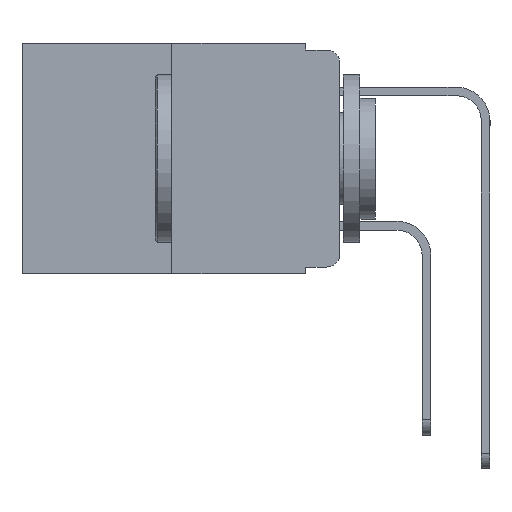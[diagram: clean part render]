
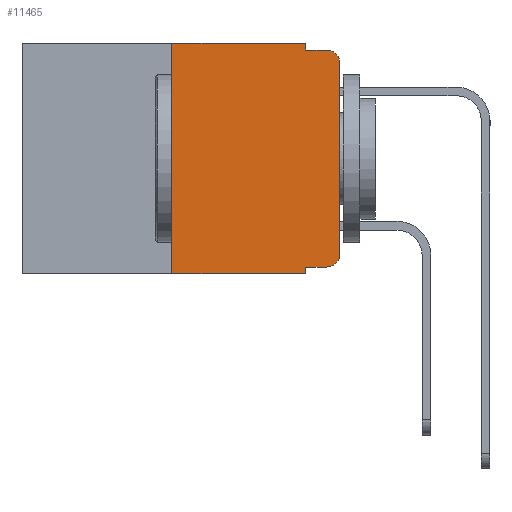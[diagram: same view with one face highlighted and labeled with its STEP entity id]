
A CAD part, left-side view. The second image highlights one B-rep face of the part: STEP entity #11465.
In plain terms, the highlighted planar face has unit normal (-1, 0, 0).
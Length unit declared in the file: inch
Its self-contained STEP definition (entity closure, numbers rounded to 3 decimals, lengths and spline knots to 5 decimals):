
#160 = CIRCLE ( 'NONE', #3296, 0.02 ) ;
#465 = LINE ( 'NONE', #10963, #16207 ) ;
#964 = VECTOR ( 'NONE', #10694, 39.37008 ) ;
#1460 = DIRECTION ( 'NONE',  ( 0., 0., -1. ) ) ;
#1743 = CARTESIAN_POINT ( 'NONE',  ( 0., 0.25, -0.343 ) ) ;
#1821 = ORIENTED_EDGE ( 'NONE', *, *, #17455, .T. ) ;
#2290 = CARTESIAN_POINT ( 'NONE',  ( 0., 0.051, -0.01 ) ) ;
#2610 = DIRECTION ( 'NONE',  ( -1., 0., 0. ) ) ;
#2672 = CARTESIAN_POINT ( 'NONE',  ( 0., 0.051, 0. ) ) ;
#2952 = VECTOR ( 'NONE', #3885, 39.37008 ) ;
#3296 = AXIS2_PLACEMENT_3D ( 'NONE', #12593, #3349, #14010 ) ;
#3349 = DIRECTION ( 'NONE',  ( -1., 0., 0. ) ) ;
#3565 = ORIENTED_EDGE ( 'NONE', *, *, #5892, .T. ) ;
#3727 = VERTEX_POINT ( 'NONE', #6033 ) ;
#3885 = DIRECTION ( 'NONE',  ( 0., -1., 0. ) ) ;
#4362 = VERTEX_POINT ( 'NONE', #10721 ) ;
#4515 = ORIENTED_EDGE ( 'NONE', *, *, #9894, .F. ) ;
#4731 = DIRECTION ( 'NONE',  ( 0., 0., -1. ) ) ;
#4883 = CARTESIAN_POINT ( 'NONE',  ( 0., 0.25, 0. ) ) ;
#4948 = CARTESIAN_POINT ( 'NONE',  ( 0., 0.051, -0.333 ) ) ;
#4962 = CARTESIAN_POINT ( 'NONE',  ( 0., 0.473, -0.343 ) ) ;
#4965 = ORIENTED_EDGE ( 'NONE', *, *, #12115, .F. ) ;
#5280 = FACE_OUTER_BOUND ( 'NONE', #14975, .T. ) ;
#5419 = ORIENTED_EDGE ( 'NONE', *, *, #14297, .F. ) ;
#5624 = VERTEX_POINT ( 'NONE', #2672 ) ;
#5887 = ORIENTED_EDGE ( 'NONE', *, *, #9923, .F. ) ;
#5892 = EDGE_CURVE ( 'NONE', #4362, #3727, #160, .T. ) ;
#6033 = CARTESIAN_POINT ( 'NONE',  ( 0., 0.02, -0.01 ) ) ;
#6136 = LINE ( 'NONE', #8270, #17377 ) ;
#6349 = ORIENTED_EDGE ( 'NONE', *, *, #9714, .T. ) ;
#6578 = VERTEX_POINT ( 'NONE', #12846 ) ;
#6692 = VECTOR ( 'NONE', #8603, 39.37008 ) ;
#6810 = ORIENTED_EDGE ( 'NONE', *, *, #8343, .F. ) ;
#6945 = LINE ( 'NONE', #4962, #14402 ) ;
#7070 = VERTEX_POINT ( 'NONE', #4883 ) ;
#7189 = ORIENTED_EDGE ( 'NONE', *, *, #17972, .T. ) ;
#7715 = VERTEX_POINT ( 'NONE', #15572 ) ;
#8114 = ORIENTED_EDGE ( 'NONE', *, *, #12686, .T. ) ;
#8270 = CARTESIAN_POINT ( 'NONE',  ( 0., 0., 0. ) ) ;
#8343 = EDGE_CURVE ( 'NONE', #10210, #6578, #16167, .T. ) ;
#8520 = VERTEX_POINT ( 'NONE', #12810 ) ;
#8603 = DIRECTION ( 'NONE',  ( 0., 0., 1. ) ) ;
#8668 = CARTESIAN_POINT ( 'NONE',  ( 0., 0.25, 0. ) ) ;
#9414 = PLANE ( 'NONE',  #11606 ) ;
#9714 = EDGE_CURVE ( 'NONE', #13393, #6578, #6945, .T. ) ;
#9894 = EDGE_CURVE ( 'NONE', #7715, #3727, #18765, .T. ) ;
#9923 = EDGE_CURVE ( 'NONE', #13393, #7070, #11293, .T. ) ;
#10210 = VERTEX_POINT ( 'NONE', #12323 ) ;
#10694 = DIRECTION ( 'NONE',  ( 0., 0., -1. ) ) ;
#10721 = CARTESIAN_POINT ( 'NONE',  ( 0., 0., -0.03 ) ) ;
#10761 = DIRECTION ( 'NONE',  ( 0., -1., 0. ) ) ;
#10928 = DIRECTION ( 'NONE',  ( 1., 0., 0. ) ) ;
#10963 = CARTESIAN_POINT ( 'NONE',  ( 0., 0.473, 0. ) ) ;
#11088 = CIRCLE ( 'NONE', #12112, 0.02 ) ;
#11286 = DIRECTION ( 'NONE',  ( 0., 0., 1. ) ) ;
#11293 = LINE ( 'NONE', #8668, #6692 ) ;
#11465 = ADVANCED_FACE ( 'NONE', ( #5280 ), #9414, .F. ) ;
#11606 = AXIS2_PLACEMENT_3D ( 'NONE', #17920, #10928, #1460 ) ;
#11953 = CARTESIAN_POINT ( 'NONE',  ( 0., 0.02, -0.313 ) ) ;
#12112 = AXIS2_PLACEMENT_3D ( 'NONE', #11953, #2610, #13364 ) ;
#12115 = EDGE_CURVE ( 'NONE', #5624, #7715, #12912, .T. ) ;
#12323 = CARTESIAN_POINT ( 'NONE',  ( 0., 0.051, -0.333 ) ) ;
#12431 = VECTOR ( 'NONE', #4731, 39.37008 ) ;
#12564 = DIRECTION ( 'NONE',  ( 0., -1., 0. ) ) ;
#12593 = CARTESIAN_POINT ( 'NONE',  ( 0., 0.02, -0.03 ) ) ;
#12686 = EDGE_CURVE ( 'NONE', #8520, #15827, #11088, .T. ) ;
#12810 = CARTESIAN_POINT ( 'NONE',  ( 0., 0.02, -0.333 ) ) ;
#12846 = CARTESIAN_POINT ( 'NONE',  ( 0., 0.051, -0.343 ) ) ;
#12912 = LINE ( 'NONE', #17708, #964 ) ;
#13364 = DIRECTION ( 'NONE',  ( 0., 0., -1. ) ) ;
#13393 = VERTEX_POINT ( 'NONE', #1743 ) ;
#14010 = DIRECTION ( 'NONE',  ( 0., 0., -1. ) ) ;
#14297 = EDGE_CURVE ( 'NONE', #7070, #5624, #465, .T. ) ;
#14402 = VECTOR ( 'NONE', #10761, 39.37008 ) ;
#14773 = LINE ( 'NONE', #4948, #18458 ) ;
#14975 = EDGE_LOOP ( 'NONE', ( #1821, #3565, #4515, #4965, #5419, #5887, #6349, #6810, #7189, #8114 ) ) ;
#15234 = DIRECTION ( 'NONE',  ( 0., -1., 0. ) ) ;
#15572 = CARTESIAN_POINT ( 'NONE',  ( 0., 0.051, -0.01 ) ) ;
#15827 = VERTEX_POINT ( 'NONE', #16166 ) ;
#16166 = CARTESIAN_POINT ( 'NONE',  ( 0., 0., -0.313 ) ) ;
#16167 = LINE ( 'NONE', #17936, #12431 ) ;
#16207 = VECTOR ( 'NONE', #15234, 39.37008 ) ;
#17377 = VECTOR ( 'NONE', #11286, 39.37008 ) ;
#17455 = EDGE_CURVE ( 'NONE', #15827, #4362, #6136, .T. ) ;
#17708 = CARTESIAN_POINT ( 'NONE',  ( 0., 0.051, 0. ) ) ;
#17920 = CARTESIAN_POINT ( 'NONE',  ( 0., 0.473, 0. ) ) ;
#17936 = CARTESIAN_POINT ( 'NONE',  ( 0., 0.051, 0. ) ) ;
#17972 = EDGE_CURVE ( 'NONE', #10210, #8520, #14773, .T. ) ;
#18458 = VECTOR ( 'NONE', #12564, 39.37008 ) ;
#18765 = LINE ( 'NONE', #2290, #2952 ) ;
